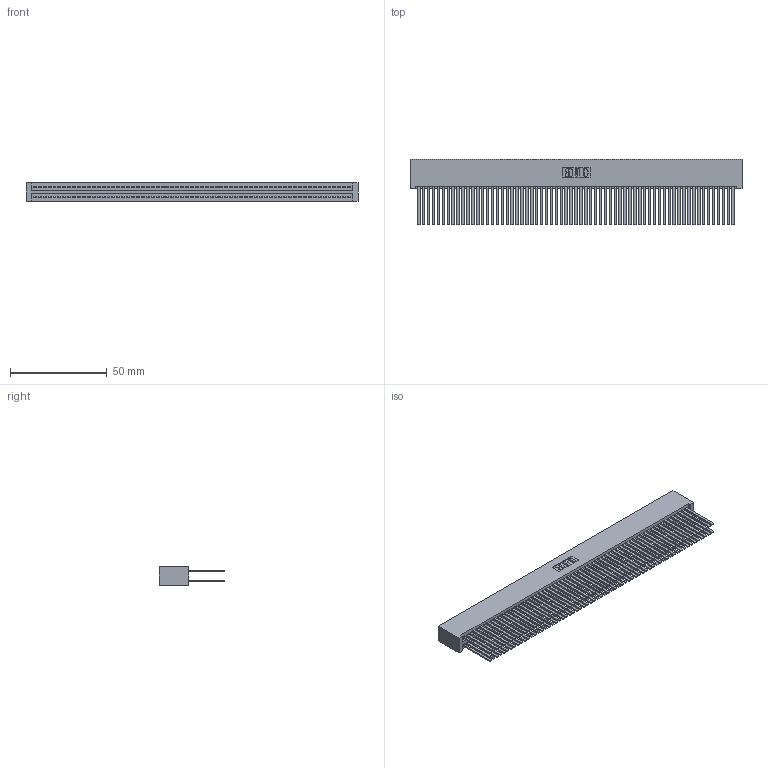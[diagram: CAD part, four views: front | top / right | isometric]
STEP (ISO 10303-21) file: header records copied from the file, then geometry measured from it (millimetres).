
FILE_DESCRIPTION (( 'STEP AP203' ), '1' );
FILE_NAME ('395-130-544-201.STEP', '2019-10-28T23:37:14', ( '' ), ( '' ), 'SwSTEP 2.0', 'SolidWorks 2016', '' );
FILE_SCHEMA (( 'CONFIG_CONTROL_DESIGN' ));
Length unit declared in the file: inch
Products named in the file (3): 345 Part_No Mounting Lugs; 345-292-001_345-293-144; 395-130-544-201
Assembly tree (131 placements, depth 2):
  395-130-544-201
    345 Part_No Mounting Lugs
    345-292-001_345-293-144  x130
Bounding box: 171.7 x 33.96 x 9.4 mm (x, y, z)
Volume: 19331.3 mm3; surface area: 34664.8 mm2
Topology: 131 solids, 131 shells, 5838 faces, 17347 edges, 11390 vertices
Faces by surface type: plane 3846, cylinder 1992
Entity records: 47443 total; most frequent: CARTESIAN_POINT 7928, ORIENTED_EDGE 7862, DIRECTION 6955, EDGE_CURVE 3931, LINE 3551, VECTOR 3551, VERTEX_POINT 2618, AXIS2_PLACEMENT_3D 1702
